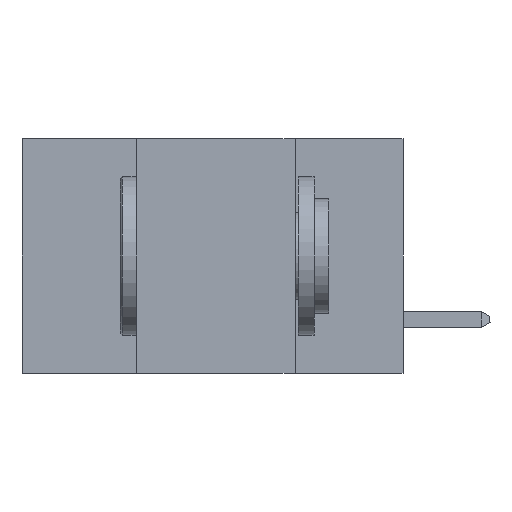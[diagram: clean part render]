
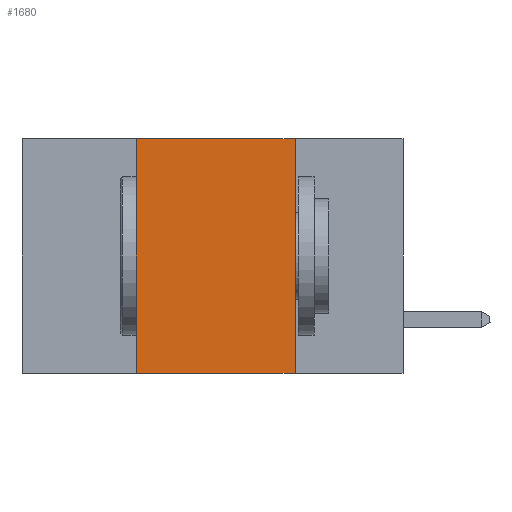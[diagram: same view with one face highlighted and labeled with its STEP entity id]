
A CAD part, left-side view. The second image highlights one B-rep face of the part: STEP entity #1680.
In plain terms, the highlighted planar face has unit normal (-1, 0, 0).
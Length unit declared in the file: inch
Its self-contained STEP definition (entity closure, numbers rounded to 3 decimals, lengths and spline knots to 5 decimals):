
#745 = VECTOR ( 'NONE', #9287, 39.37008 ) ;
#926 = CARTESIAN_POINT ( 'NONE',  ( 0., 0.17, 0. ) ) ;
#1011 = CARTESIAN_POINT ( 'NONE',  ( 0., 0.42, 0. ) ) ;
#1294 = CARTESIAN_POINT ( 'NONE',  ( 0., 0.6, -0.37 ) ) ;
#1618 = CARTESIAN_POINT ( 'NONE',  ( 0., 0.17, -0.37 ) ) ;
#1680 = ADVANCED_FACE ( 'NONE', ( #5203 ), #11129, .F. ) ;
#2294 = VECTOR ( 'NONE', #4841, 39.37008 ) ;
#2349 = CARTESIAN_POINT ( 'NONE',  ( 0., 0.6, 0. ) ) ;
#3185 = DIRECTION ( 'NONE',  ( 0., 0., 1. ) ) ;
#3367 = VERTEX_POINT ( 'NONE', #926 ) ;
#3448 = DIRECTION ( 'NONE',  ( 0., 0., -1. ) ) ;
#3492 = LINE ( 'NONE', #7484, #3647 ) ;
#3647 = VECTOR ( 'NONE', #3185, 39.37008 ) ;
#3658 = VERTEX_POINT ( 'NONE', #1618 ) ;
#3840 = LINE ( 'NONE', #7287, #9620 ) ;
#4106 = EDGE_CURVE ( 'NONE', #6381, #3367, #3840, .T. ) ;
#4145 = LINE ( 'NONE', #1294, #745 ) ;
#4841 = DIRECTION ( 'NONE',  ( 0., 0., -1. ) ) ;
#5203 = FACE_OUTER_BOUND ( 'NONE', #5690, .T. ) ;
#5601 = EDGE_CURVE ( 'NONE', #3367, #3658, #6948, .T. ) ;
#5690 = EDGE_LOOP ( 'NONE', ( #10443, #9717, #6778, #7473 ) ) ;
#5771 = CARTESIAN_POINT ( 'NONE',  ( 0., 0.17, 0. ) ) ;
#5876 = DIRECTION ( 'NONE',  ( 1., 0., 0. ) ) ;
#6003 = EDGE_CURVE ( 'NONE', #10136, #6381, #3492, .T. ) ;
#6381 = VERTEX_POINT ( 'NONE', #1011 ) ;
#6405 = DIRECTION ( 'NONE',  ( 0., -1., 0. ) ) ;
#6778 = ORIENTED_EDGE ( 'NONE', *, *, #6003, .F. ) ;
#6948 = LINE ( 'NONE', #5771, #2294 ) ;
#7266 = EDGE_CURVE ( 'NONE', #10136, #3658, #4145, .T. ) ;
#7287 = CARTESIAN_POINT ( 'NONE',  ( 0., 0.6, 0. ) ) ;
#7473 = ORIENTED_EDGE ( 'NONE', *, *, #7266, .T. ) ;
#7484 = CARTESIAN_POINT ( 'NONE',  ( 0., 0.42, 0. ) ) ;
#9287 = DIRECTION ( 'NONE',  ( 0., -1., 0. ) ) ;
#9620 = VECTOR ( 'NONE', #6405, 39.37008 ) ;
#9717 = ORIENTED_EDGE ( 'NONE', *, *, #4106, .F. ) ;
#9918 = AXIS2_PLACEMENT_3D ( 'NONE', #2349, #5876, #3448 ) ;
#10136 = VERTEX_POINT ( 'NONE', #11354 ) ;
#10443 = ORIENTED_EDGE ( 'NONE', *, *, #5601, .F. ) ;
#11129 = PLANE ( 'NONE',  #9918 ) ;
#11354 = CARTESIAN_POINT ( 'NONE',  ( 0., 0.42, -0.37 ) ) ;
